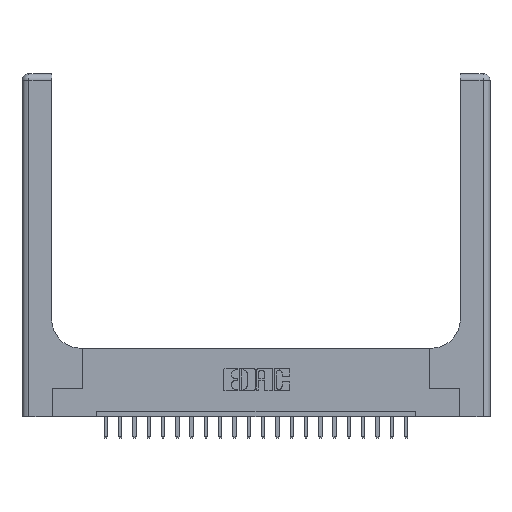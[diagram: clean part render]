
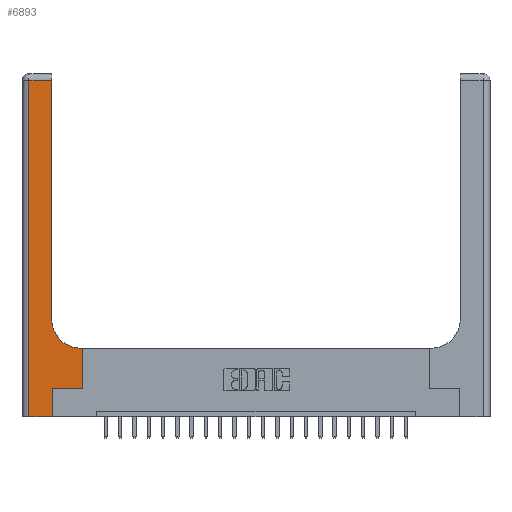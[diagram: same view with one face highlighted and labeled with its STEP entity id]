
A CAD part, top view. The second image highlights one B-rep face of the part: STEP entity #6893.
In plain terms, the highlighted planar face has unit normal (0, 0, 1).
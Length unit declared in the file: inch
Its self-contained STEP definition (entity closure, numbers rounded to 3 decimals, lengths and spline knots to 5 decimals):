
#237 = CARTESIAN_POINT ( 'NONE',  ( 0.06, 2.94, 0.37 ) ) ;
#1302 = VECTOR ( 'NONE', #10179, 39.37008 ) ;
#1381 = VERTEX_POINT ( 'NONE', #237 ) ;
#1710 = CARTESIAN_POINT ( 'NONE',  ( 0., 2.94, 0.37 ) ) ;
#1792 = DIRECTION ( 'NONE',  ( 0., 1., 0. ) ) ;
#1871 = CARTESIAN_POINT ( 'NONE',  ( 0.528, 0.25, 0.37 ) ) ;
#1887 = CARTESIAN_POINT ( 'NONE',  ( 0.26, 0.6, 0.37 ) ) ;
#2504 = VECTOR ( 'NONE', #10115, 39.37008 ) ;
#3068 = LINE ( 'NONE', #1871, #11439 ) ;
#3388 = EDGE_CURVE ( 'NONE', #1381, #8874, #6270, .T. ) ;
#3431 = CARTESIAN_POINT ( 'NONE',  ( 0.06, 0., 0.37 ) ) ;
#3920 = DIRECTION ( 'NONE',  ( 1., 0., 0. ) ) ;
#4108 = DIRECTION ( 'NONE',  ( -1., 0., 0. ) ) ;
#4448 = AXIS2_PLACEMENT_3D ( 'NONE', #14124, #17891, #21130 ) ;
#4567 = LINE ( 'NONE', #1710, #2504 ) ;
#4750 = DIRECTION ( 'NONE',  ( 0., 0., -1. ) ) ;
#4886 = CARTESIAN_POINT ( 'NONE',  ( 0.51, 0.6, 0.37 ) ) ;
#5415 = ORIENTED_EDGE ( 'NONE', *, *, #3388, .T. ) ;
#5460 = CIRCLE ( 'NONE', #10648, 0.25 ) ;
#6108 = VERTEX_POINT ( 'NONE', #6165 ) ;
#6165 = CARTESIAN_POINT ( 'NONE',  ( 0.26, 2.94, 0.37 ) ) ;
#6183 = VERTEX_POINT ( 'NONE', #4886 ) ;
#6270 = LINE ( 'NONE', #9753, #1302 ) ;
#6443 = LINE ( 'NONE', #13941, #19244 ) ;
#6674 = CARTESIAN_POINT ( 'NONE',  ( 0.26, 0.85, 0.37 ) ) ;
#6812 = VERTEX_POINT ( 'NONE', #10602 ) ;
#6893 = ADVANCED_FACE ( 'NONE', ( #12781 ), #12801, .F. ) ;
#7119 = DIRECTION ( 'NONE',  ( 1., 0., 0. ) ) ;
#7512 = ORIENTED_EDGE ( 'NONE', *, *, #15000, .T. ) ;
#8155 = CARTESIAN_POINT ( 'NONE',  ( 0.528, 0.6, 0.37 ) ) ;
#8505 = ORIENTED_EDGE ( 'NONE', *, *, #18287, .T. ) ;
#8619 = ORIENTED_EDGE ( 'NONE', *, *, #16444, .T. ) ;
#8874 = VERTEX_POINT ( 'NONE', #3431 ) ;
#9193 = EDGE_CURVE ( 'NONE', #6183, #9261, #5460, .T. ) ;
#9261 = VERTEX_POINT ( 'NONE', #6674 ) ;
#9748 = VECTOR ( 'NONE', #15657, 39.37008 ) ;
#9753 = CARTESIAN_POINT ( 'NONE',  ( 0.06, 3., 0.37 ) ) ;
#9810 = VERTEX_POINT ( 'NONE', #21327 ) ;
#9968 = EDGE_LOOP ( 'NONE', ( #19993, #16176, #5415, #8619, #8505, #13242, #7512, #20777, #17066 ) ) ;
#10057 = DIRECTION ( 'NONE',  ( 0., 1., 0. ) ) ;
#10115 = DIRECTION ( 'NONE',  ( -1., 0., 0. ) ) ;
#10179 = DIRECTION ( 'NONE',  ( 0., -1., 0. ) ) ;
#10599 = CARTESIAN_POINT ( 'NONE',  ( 0.265, 0., 0.37 ) ) ;
#10602 = CARTESIAN_POINT ( 'NONE',  ( 0.265, 0., 0.37 ) ) ;
#10621 = VECTOR ( 'NONE', #1792, 39.37008 ) ;
#10648 = AXIS2_PLACEMENT_3D ( 'NONE', #14732, #4750, #11501 ) ;
#11439 = VECTOR ( 'NONE', #10057, 39.37008 ) ;
#11501 = DIRECTION ( 'NONE',  ( 1., 0., 0. ) ) ;
#12211 = LINE ( 'NONE', #15241, #18454 ) ;
#12781 = FACE_OUTER_BOUND ( 'NONE', #9968, .T. ) ;
#12801 = PLANE ( 'NONE',  #4448 ) ;
#12973 = LINE ( 'NONE', #18492, #10621 ) ;
#13242 = ORIENTED_EDGE ( 'NONE', *, *, #15225, .T. ) ;
#13344 = LINE ( 'NONE', #1887, #14934 ) ;
#13941 = CARTESIAN_POINT ( 'NONE',  ( 0., 0., 0.37 ) ) ;
#14044 = EDGE_CURVE ( 'NONE', #6108, #1381, #4567, .T. ) ;
#14124 = CARTESIAN_POINT ( 'NONE',  ( 0., 3., 0.37 ) ) ;
#14732 = CARTESIAN_POINT ( 'NONE',  ( 0.51, 0.85, 0.37 ) ) ;
#14934 = VECTOR ( 'NONE', #4108, 39.37008 ) ;
#14970 = VERTEX_POINT ( 'NONE', #8155 ) ;
#15000 = EDGE_CURVE ( 'NONE', #9810, #14970, #3068, .T. ) ;
#15225 = EDGE_CURVE ( 'NONE', #20070, #9810, #12211, .T. ) ;
#15241 = CARTESIAN_POINT ( 'NONE',  ( 0.265, 0.25, 0.37 ) ) ;
#15657 = DIRECTION ( 'NONE',  ( 0., 1., 0. ) ) ;
#16176 = ORIENTED_EDGE ( 'NONE', *, *, #14044, .T. ) ;
#16444 = EDGE_CURVE ( 'NONE', #8874, #6812, #6443, .T. ) ;
#17066 = ORIENTED_EDGE ( 'NONE', *, *, #9193, .T. ) ;
#17578 = LINE ( 'NONE', #10599, #9748 ) ;
#17891 = DIRECTION ( 'NONE',  ( 0., 0., -1. ) ) ;
#18287 = EDGE_CURVE ( 'NONE', #6812, #20070, #17578, .T. ) ;
#18454 = VECTOR ( 'NONE', #7119, 39.37008 ) ;
#18492 = CARTESIAN_POINT ( 'NONE',  ( 0.26, 3., 0.37 ) ) ;
#19244 = VECTOR ( 'NONE', #3920, 39.37008 ) ;
#19547 = EDGE_CURVE ( 'NONE', #14970, #6183, #13344, .T. ) ;
#19993 = ORIENTED_EDGE ( 'NONE', *, *, #20906, .T. ) ;
#20027 = CARTESIAN_POINT ( 'NONE',  ( 0.265, 0.25, 0.37 ) ) ;
#20070 = VERTEX_POINT ( 'NONE', #20027 ) ;
#20777 = ORIENTED_EDGE ( 'NONE', *, *, #19547, .T. ) ;
#20906 = EDGE_CURVE ( 'NONE', #9261, #6108, #12973, .T. ) ;
#21130 = DIRECTION ( 'NONE',  ( -1., 0., 0. ) ) ;
#21327 = CARTESIAN_POINT ( 'NONE',  ( 0.528, 0.25, 0.37 ) ) ;
